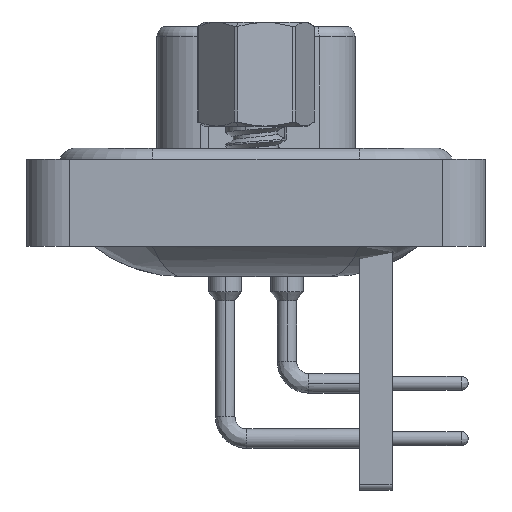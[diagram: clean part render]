
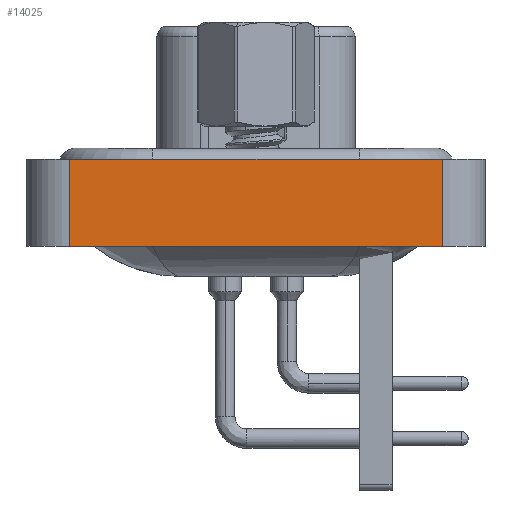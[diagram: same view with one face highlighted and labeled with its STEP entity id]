
A CAD part, left-side view. The second image highlights one B-rep face of the part: STEP entity #14025.
In plain terms, the highlighted planar face has unit normal (-1, 0, 0).
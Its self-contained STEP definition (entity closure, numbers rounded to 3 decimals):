
#271 = LINE ( 'NONE', #2107, #20796 ) ;
#571 = EDGE_CURVE ( 'NONE', #3129, #10036, #271, .T. ) ;
#941 = CARTESIAN_POINT ( 'NONE',  ( -7.26, -8.55, 0.4 ) ) ;
#1181 = EDGE_LOOP ( 'NONE', ( #1608, #24944, #18121, #10069 ) ) ;
#1608 = ORIENTED_EDGE ( 'NONE', *, *, #20350, .T. ) ;
#2107 = CARTESIAN_POINT ( 'NONE',  ( -7.26, -8.55, -3.6 ) ) ;
#3129 = VERTEX_POINT ( 'NONE', #11555 ) ;
#4820 = DIRECTION ( 'NONE',  ( -1., 0., 0. ) ) ;
#5160 = CARTESIAN_POINT ( 'NONE',  ( -7.26, -8.55, 0.4 ) ) ;
#5233 = DIRECTION ( 'NONE',  ( 0., 0., 1. ) ) ;
#10036 = VERTEX_POINT ( 'NONE', #13748 ) ;
#10069 = ORIENTED_EDGE ( 'NONE', *, *, #571, .T. ) ;
#10070 = VECTOR ( 'NONE', #5233, 1000. ) ;
#10233 = LINE ( 'NONE', #22529, #25005 ) ;
#10794 = PLANE ( 'NONE',  #11137 ) ;
#11137 = AXIS2_PLACEMENT_3D ( 'NONE', #15140, #4820, #22698 ) ;
#11555 = CARTESIAN_POINT ( 'NONE',  ( -7.26, 8.55, -3.6 ) ) ;
#12574 = DIRECTION ( 'NONE',  ( 0., -1., 0. ) ) ;
#13748 = CARTESIAN_POINT ( 'NONE',  ( -7.26, -8.55, -3.6 ) ) ;
#14025 = ADVANCED_FACE ( 'NONE', ( #14622 ), #10794, .T. ) ;
#14622 = FACE_OUTER_BOUND ( 'NONE', #1181, .T. ) ;
#14730 = VERTEX_POINT ( 'NONE', #941 ) ;
#15140 = CARTESIAN_POINT ( 'NONE',  ( -7.26, -8.55, -3.6 ) ) ;
#15301 = CARTESIAN_POINT ( 'NONE',  ( -7.26, 8.55, -3.6 ) ) ;
#15503 = VERTEX_POINT ( 'NONE', #16434 ) ;
#16434 = CARTESIAN_POINT ( 'NONE',  ( -7.26, 8.55, 0.4 ) ) ;
#16888 = LINE ( 'NONE', #15301, #10070 ) ;
#18121 = ORIENTED_EDGE ( 'NONE', *, *, #26155, .F. ) ;
#19226 = VECTOR ( 'NONE', #21447, 1000. ) ;
#19323 = LINE ( 'NONE', #5160, #19226 ) ;
#20350 = EDGE_CURVE ( 'NONE', #10036, #14730, #10233, .T. ) ;
#20796 = VECTOR ( 'NONE', #12574, 1000. ) ;
#20805 = DIRECTION ( 'NONE',  ( 0., 0., 1. ) ) ;
#21447 = DIRECTION ( 'NONE',  ( 0., -1., 0. ) ) ;
#22529 = CARTESIAN_POINT ( 'NONE',  ( -7.26, -8.55, -3.6 ) ) ;
#22698 = DIRECTION ( 'NONE',  ( 0., 0., 1. ) ) ;
#24510 = EDGE_CURVE ( 'NONE', #15503, #14730, #19323, .T. ) ;
#24944 = ORIENTED_EDGE ( 'NONE', *, *, #24510, .F. ) ;
#25005 = VECTOR ( 'NONE', #20805, 1000. ) ;
#26155 = EDGE_CURVE ( 'NONE', #3129, #15503, #16888, .T. ) ;
